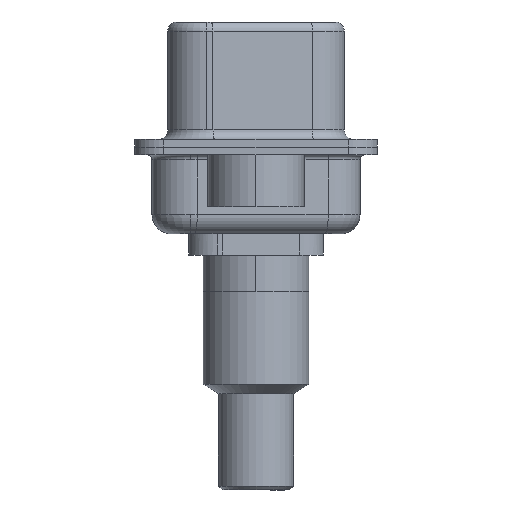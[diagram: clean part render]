
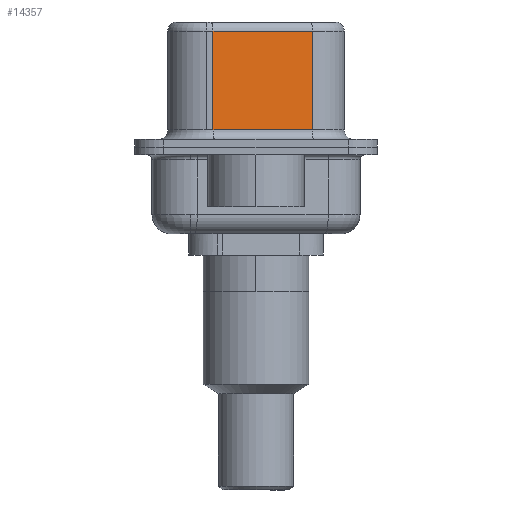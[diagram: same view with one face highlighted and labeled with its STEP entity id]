
A CAD part, left-side view. The second image highlights one B-rep face of the part: STEP entity #14357.
In plain terms, the highlighted planar face has unit normal (-0.985, -0.174, 0).
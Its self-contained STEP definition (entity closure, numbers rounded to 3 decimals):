
#690 = EDGE_CURVE ( 'NONE', #6864, #22335, #21403, .T. ) ;
#1033 = VECTOR ( 'NONE', #18438, 1000. ) ;
#1976 = CARTESIAN_POINT ( 'NONE',  ( 3.675, 2.233, 6.52 ) ) ;
#2140 = EDGE_CURVE ( 'NONE', #6864, #21657, #16776, .T. ) ;
#2924 = EDGE_CURVE ( 'NONE', #21657, #17258, #9035, .T. ) ;
#3772 = VECTOR ( 'NONE', #15645, 1000. ) ;
#6308 = VECTOR ( 'NONE', #9094, 1000. ) ;
#6604 = EDGE_LOOP ( 'NONE', ( #22547, #13541, #12515, #17999 ) ) ;
#6864 = VERTEX_POINT ( 'NONE', #9917 ) ;
#6872 = FACE_OUTER_BOUND ( 'NONE', #6604, .T. ) ;
#7162 = CARTESIAN_POINT ( 'NONE',  ( 4.585, -2.927, 6.52 ) ) ;
#7804 = VECTOR ( 'NONE', #25393, 1000. ) ;
#9035 = LINE ( 'NONE', #1976, #3772 ) ;
#9094 = DIRECTION ( 'NONE',  ( 0., 0., -1. ) ) ;
#9145 = DIRECTION ( 'NONE',  ( 0.985, 0.174, 0. ) ) ;
#9798 = AXIS2_PLACEMENT_3D ( 'NONE', #7162, #9145, #22935 ) ;
#9917 = CARTESIAN_POINT ( 'NONE',  ( 4.585, -2.927, 6.02 ) ) ;
#11108 = CARTESIAN_POINT ( 'NONE',  ( 4.585, -2.927, 6.52 ) ) ;
#12515 = ORIENTED_EDGE ( 'NONE', *, *, #2924, .T. ) ;
#13168 = CARTESIAN_POINT ( 'NONE',  ( 3.675, 2.233, 0.9 ) ) ;
#13541 = ORIENTED_EDGE ( 'NONE', *, *, #2140, .T. ) ;
#14357 = ADVANCED_FACE ( 'NONE', ( #6872 ), #19007, .F. ) ;
#14529 = EDGE_CURVE ( 'NONE', #17258, #22335, #18306, .T. ) ;
#15645 = DIRECTION ( 'NONE',  ( 0., 0., -1. ) ) ;
#16776 = LINE ( 'NONE', #18099, #1033 ) ;
#17258 = VERTEX_POINT ( 'NONE', #13168 ) ;
#17526 = CARTESIAN_POINT ( 'NONE',  ( 4.585, -2.927, 0.9 ) ) ;
#17999 = ORIENTED_EDGE ( 'NONE', *, *, #14529, .T. ) ;
#18099 = CARTESIAN_POINT ( 'NONE',  ( 4.585, -2.927, 6.02 ) ) ;
#18306 = LINE ( 'NONE', #17526, #7804 ) ;
#18438 = DIRECTION ( 'NONE',  ( -0.174, 0.985, 0. ) ) ;
#19007 = PLANE ( 'NONE',  #9798 ) ;
#20888 = CARTESIAN_POINT ( 'NONE',  ( 4.585, -2.927, 0.9 ) ) ;
#21093 = CARTESIAN_POINT ( 'NONE',  ( 3.675, 2.233, 6.02 ) ) ;
#21403 = LINE ( 'NONE', #11108, #6308 ) ;
#21657 = VERTEX_POINT ( 'NONE', #21093 ) ;
#22335 = VERTEX_POINT ( 'NONE', #20888 ) ;
#22547 = ORIENTED_EDGE ( 'NONE', *, *, #690, .F. ) ;
#22935 = DIRECTION ( 'NONE',  ( -0.174, 0.985, 0. ) ) ;
#25393 = DIRECTION ( 'NONE',  ( 0.174, -0.985, 0. ) ) ;
